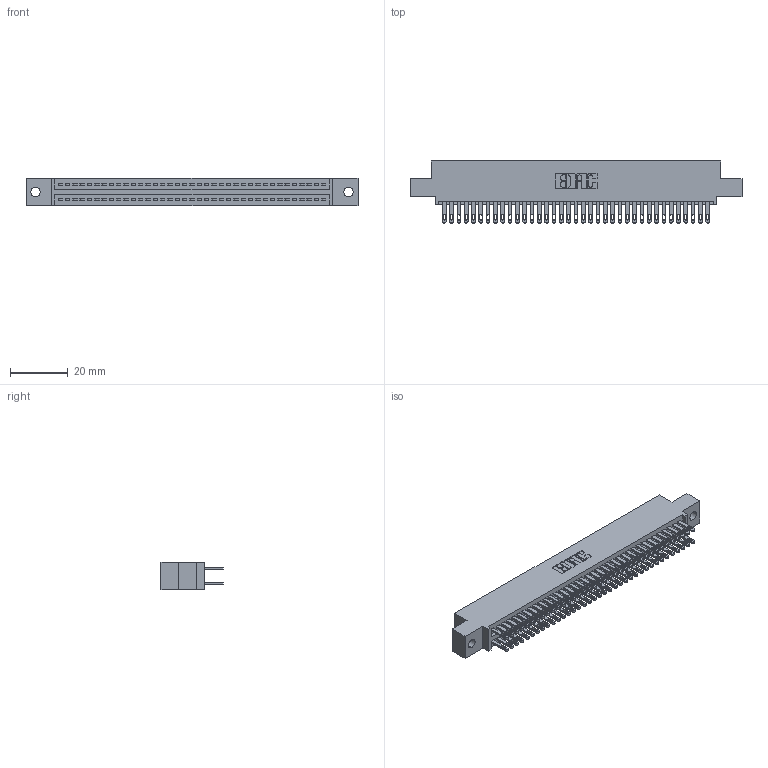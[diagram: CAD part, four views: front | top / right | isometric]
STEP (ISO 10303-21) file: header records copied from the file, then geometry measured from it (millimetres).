
FILE_DESCRIPTION (( 'STEP AP203' ), '1' );
FILE_NAME ('345-074-500-502.STEP', '2019-10-31T05:25:42', ( '' ), ( '' ), 'SwSTEP 2.0', 'SolidWorks 2016', '' );
FILE_SCHEMA (( 'CONFIG_CONTROL_DESIGN' ));
Length unit declared in the file: inch
Products named in the file (3): 345 Part_0.110 Offset - 0.128 Dia; 345-292-001_345-293-100; 345-074-500-502
Assembly tree (75 placements, depth 2):
  345-074-500-502
    345 Part_0.110 Offset - 0.128 Dia
    345-292-001_345-293-100  x74
Bounding box: 115.19 x 21.51 x 9.4 mm (x, y, z)
Volume: 11259.2 mm3; surface area: 17121.1 mm2
Topology: 75 solids, 75 shells, 3534 faces, 10787 edges, 7190 vertices
Faces by surface type: plane 2082, cylinder 1452
Entity records: 29769 total; most frequent: CARTESIAN_POINT 4996, ORIENTED_EDGE 4930, DIRECTION 4413, EDGE_CURVE 2465, VECTOR 2181, LINE 2181, VERTEX_POINT 1642, AXIS2_PLACEMENT_3D 1116
